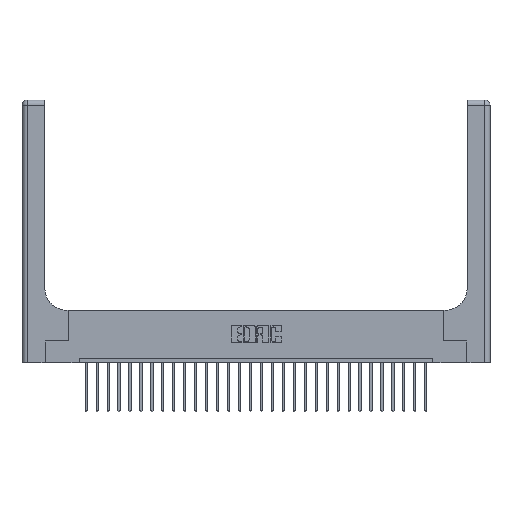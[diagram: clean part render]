
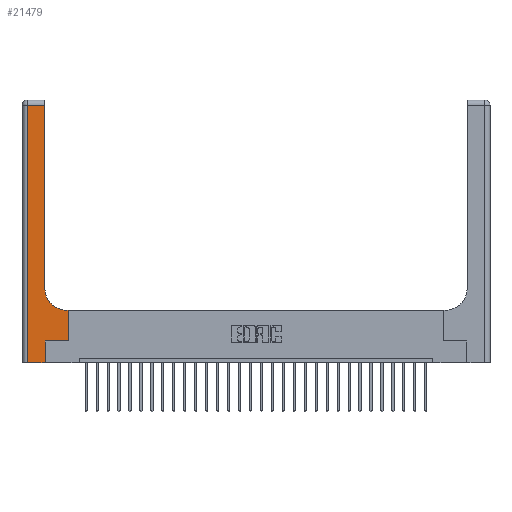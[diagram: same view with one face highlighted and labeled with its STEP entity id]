
A CAD part, top view. The second image highlights one B-rep face of the part: STEP entity #21479.
In plain terms, the highlighted planar face has unit normal (0, 0, 1).
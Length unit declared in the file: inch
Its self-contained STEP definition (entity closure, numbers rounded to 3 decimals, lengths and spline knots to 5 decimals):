
#194 = ORIENTED_EDGE ( 'NONE', *, *, #10613, .T. ) ;
#833 = ORIENTED_EDGE ( 'NONE', *, *, #1544, .T. ) ;
#985 = ORIENTED_EDGE ( 'NONE', *, *, #4817, .T. ) ;
#1196 = DIRECTION ( 'NONE',  ( -1., 0., 0. ) ) ;
#1544 = EDGE_CURVE ( 'NONE', #17447, #5562, #26262, .T. ) ;
#1637 = CARTESIAN_POINT ( 'NONE',  ( 0., 0., 0.37 ) ) ;
#1785 = VECTOR ( 'NONE', #5987, 39.37008 ) ;
#3189 = VERTEX_POINT ( 'NONE', #17622 ) ;
#3685 = LINE ( 'NONE', #1637, #1785 ) ;
#4208 = CARTESIAN_POINT ( 'NONE',  ( 0.265, 0.25, 0.37 ) ) ;
#4317 = CARTESIAN_POINT ( 'NONE',  ( 0.26, 0.6, 0.37 ) ) ;
#4409 = CARTESIAN_POINT ( 'NONE',  ( 0.26, 3., 0.37 ) ) ;
#4512 = EDGE_CURVE ( 'NONE', #26683, #3189, #23880, .T. ) ;
#4817 = EDGE_CURVE ( 'NONE', #7076, #17447, #6231, .T. ) ;
#5562 = VERTEX_POINT ( 'NONE', #20145 ) ;
#5738 = ORIENTED_EDGE ( 'NONE', *, *, #26388, .T. ) ;
#5987 = DIRECTION ( 'NONE',  ( 1., 0., 0. ) ) ;
#6231 = LINE ( 'NONE', #8788, #19535 ) ;
#6695 = DIRECTION ( 'NONE',  ( 1., 0., 0. ) ) ;
#7076 = VERTEX_POINT ( 'NONE', #8645 ) ;
#7380 = DIRECTION ( 'NONE',  ( 1., 0., 0. ) ) ;
#7621 = CARTESIAN_POINT ( 'NONE',  ( 0.26, 0.85, 0.37 ) ) ;
#8027 = VECTOR ( 'NONE', #20357, 39.37008 ) ;
#8199 = VECTOR ( 'NONE', #16891, 39.37008 ) ;
#8384 = LINE ( 'NONE', #4317, #16454 ) ;
#8540 = ORIENTED_EDGE ( 'NONE', *, *, #21250, .T. ) ;
#8645 = CARTESIAN_POINT ( 'NONE',  ( 0.265, 0., 0.37 ) ) ;
#8671 = PLANE ( 'NONE',  #10810 ) ;
#8788 = CARTESIAN_POINT ( 'NONE',  ( 0.265, 0., 0.37 ) ) ;
#9924 = CIRCLE ( 'NONE', #13375, 0.25 ) ;
#10106 = ORIENTED_EDGE ( 'NONE', *, *, #4512, .T. ) ;
#10207 = EDGE_CURVE ( 'NONE', #16872, #7076, #3685, .T. ) ;
#10386 = CARTESIAN_POINT ( 'NONE',  ( 0.26, 2.94, 0.37 ) ) ;
#10613 = EDGE_CURVE ( 'NONE', #3189, #16872, #24426, .T. ) ;
#10810 = AXIS2_PLACEMENT_3D ( 'NONE', #19250, #22947, #25088 ) ;
#11670 = ORIENTED_EDGE ( 'NONE', *, *, #17325, .T. ) ;
#11690 = LINE ( 'NONE', #18057, #17650 ) ;
#11815 = DIRECTION ( 'NONE',  ( 0., 0., -1. ) ) ;
#12102 = VECTOR ( 'NONE', #1196, 39.37008 ) ;
#13130 = VERTEX_POINT ( 'NONE', #7621 ) ;
#13375 = AXIS2_PLACEMENT_3D ( 'NONE', #13835, #11815, #6695 ) ;
#13502 = ORIENTED_EDGE ( 'NONE', *, *, #10207, .T. ) ;
#13835 = CARTESIAN_POINT ( 'NONE',  ( 0.51, 0.85, 0.37 ) ) ;
#16454 = VECTOR ( 'NONE', #22926, 39.37008 ) ;
#16686 = EDGE_LOOP ( 'NONE', ( #17203, #10106, #194, #13502, #985, #833, #11670, #5738, #8540 ) ) ;
#16872 = VERTEX_POINT ( 'NONE', #18112 ) ;
#16891 = DIRECTION ( 'NONE',  ( 0., 1., 0. ) ) ;
#17203 = ORIENTED_EDGE ( 'NONE', *, *, #21094, .T. ) ;
#17325 = EDGE_CURVE ( 'NONE', #5562, #23628, #11690, .T. ) ;
#17447 = VERTEX_POINT ( 'NONE', #4208 ) ;
#17622 = CARTESIAN_POINT ( 'NONE',  ( 0.06, 2.94, 0.37 ) ) ;
#17650 = VECTOR ( 'NONE', #26340, 39.37008 ) ;
#17783 = CARTESIAN_POINT ( 'NONE',  ( 0.06, 3., 0.37 ) ) ;
#17929 = CARTESIAN_POINT ( 'NONE',  ( 0.528, 0.6, 0.37 ) ) ;
#18057 = CARTESIAN_POINT ( 'NONE',  ( 0.528, 0.25, 0.37 ) ) ;
#18112 = CARTESIAN_POINT ( 'NONE',  ( 0.06, 0., 0.37 ) ) ;
#18693 = CARTESIAN_POINT ( 'NONE',  ( 0.51, 0.6, 0.37 ) ) ;
#19250 = CARTESIAN_POINT ( 'NONE',  ( 0., 3., 0.37 ) ) ;
#19394 = CARTESIAN_POINT ( 'NONE',  ( 0., 2.94, 0.37 ) ) ;
#19535 = VECTOR ( 'NONE', #21028, 39.37008 ) ;
#20145 = CARTESIAN_POINT ( 'NONE',  ( 0.528, 0.25, 0.37 ) ) ;
#20357 = DIRECTION ( 'NONE',  ( 0., -1., 0. ) ) ;
#20658 = VERTEX_POINT ( 'NONE', #18693 ) ;
#21028 = DIRECTION ( 'NONE',  ( 0., 1., 0. ) ) ;
#21094 = EDGE_CURVE ( 'NONE', #13130, #26683, #24887, .T. ) ;
#21250 = EDGE_CURVE ( 'NONE', #20658, #13130, #9924, .T. ) ;
#21479 = ADVANCED_FACE ( 'NONE', ( #25221 ), #8671, .F. ) ;
#22926 = DIRECTION ( 'NONE',  ( -1., 0., 0. ) ) ;
#22947 = DIRECTION ( 'NONE',  ( 0., 0., -1. ) ) ;
#23390 = VECTOR ( 'NONE', #7380, 39.37008 ) ;
#23628 = VERTEX_POINT ( 'NONE', #17929 ) ;
#23880 = LINE ( 'NONE', #19394, #12102 ) ;
#24426 = LINE ( 'NONE', #17783, #8027 ) ;
#24887 = LINE ( 'NONE', #4409, #8199 ) ;
#25088 = DIRECTION ( 'NONE',  ( -1., 0., 0. ) ) ;
#25221 = FACE_OUTER_BOUND ( 'NONE', #16686, .T. ) ;
#26262 = LINE ( 'NONE', #26400, #23390 ) ;
#26340 = DIRECTION ( 'NONE',  ( 0., 1., 0. ) ) ;
#26388 = EDGE_CURVE ( 'NONE', #23628, #20658, #8384, .T. ) ;
#26400 = CARTESIAN_POINT ( 'NONE',  ( 0.265, 0.25, 0.37 ) ) ;
#26683 = VERTEX_POINT ( 'NONE', #10386 ) ;
